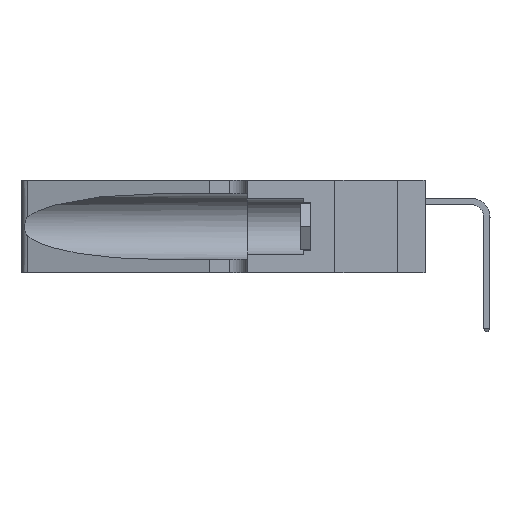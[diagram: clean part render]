
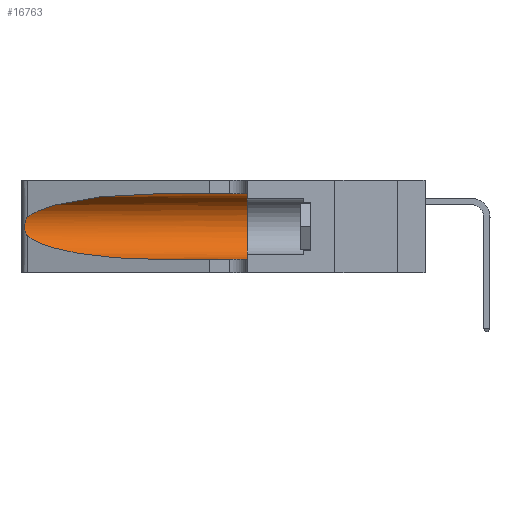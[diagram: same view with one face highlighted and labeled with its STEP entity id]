
A CAD part, left-side view. The second image highlights one B-rep face of the part: STEP entity #16763.
In plain terms, the highlighted cylindrical face has radius 3.308 mm (diameter 6.617 mm), a partial arc.
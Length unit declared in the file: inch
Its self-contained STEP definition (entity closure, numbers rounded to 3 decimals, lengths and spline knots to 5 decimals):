
#260 = CARTESIAN_POINT ( 'NONE',  ( 0.1305, 0.72297, 0.31525 ) ) ;
#301 = CARTESIAN_POINT ( 'NONE',  ( 0.25487, 1.22718, 0.14631 ) ) ;
#3483 = CARTESIAN_POINT ( 'NONE',  ( 0.25639, 1.23184, 0.21858 ) ) ;
#4740 = VERTEX_POINT ( 'NONE', #5156 ) ;
#5156 = CARTESIAN_POINT ( 'NONE',  ( 0.1305, 0.35, 0.31525 ) ) ;
#5335 = LINE ( 'NONE', #23273, #21573 ) ;
#6821 = CARTESIAN_POINT ( 'NONE',  ( 0.25854, 1.2359, 0.20912 ) ) ;
#8259 = EDGE_CURVE ( 'NONE', #13565, #40154, #20886, .T. ) ;
#8665 = CARTESIAN_POINT ( 'NONE',  ( 0.25487, 1.22718, 0.14631 ) ) ;
#10101 = CARTESIAN_POINT ( 'NONE',  ( 0.26075, 1.23896, 0.19203 ) ) ;
#10343 = EDGE_CURVE ( 'NONE', #40500, #4740, #37743, .T. ) ;
#13371 = CARTESIAN_POINT ( 'NONE',  ( 0.26017, 1.23833, 0.17102 ) ) ;
#13480 = CYLINDRICAL_SURFACE ( 'NONE', #17492, 0.13025 ) ;
#13565 = VERTEX_POINT ( 'NONE', #40414 ) ;
#14481 = FACE_OUTER_BOUND ( 'NONE', #26450, .T. ) ;
#14587 = DIRECTION ( 'NONE',  ( 0., 0., -1. ) ) ;
#14667 = CARTESIAN_POINT ( 'NONE',  ( 0.1305, 0.72297, 0.31525 ) ) ;
#15655 = CARTESIAN_POINT ( 'NONE',  ( 0.25487, 1.22718, 0.22369 ) ) ;
#16059 = ORIENTED_EDGE ( 'NONE', *, *, #21133, .T. ) ;
#16588 = CARTESIAN_POINT ( 'NONE',  ( 0.25789, 1.23486, 0.15765 ) ) ;
#16763 = ADVANCED_FACE ( 'NONE', ( #14481 ), #13480, .F. ) ;
#17492 = AXIS2_PLACEMENT_3D ( 'NONE', #21084, #37221, #14587 ) ;
#17765 = CARTESIAN_POINT ( 'NONE',  ( 0.18966, 0.96281, 0.31525 ) ) ;
#18184 = ORIENTED_EDGE ( 'NONE', *, *, #8259, .T. ) ;
#18957 = EDGE_CURVE ( 'NONE', #4740, #27618, #39060, .T. ) ;
#19145 = CARTESIAN_POINT ( 'NONE',  ( 0.1305, 0.35, 0.185 ) ) ;
#19700 = CARTESIAN_POINT ( 'NONE',  ( 0.25487, 1.22718, 0.22369 ) ) ;
#19837 = CARTESIAN_POINT ( 'NONE',  ( 0.25555, 1.22993, 0.14849 ) ) ;
#20022 = DIRECTION ( 'NONE',  ( 0., -1., 0. ) ) ;
#20886 =( BOUNDED_CURVE ( )  B_SPLINE_CURVE ( 3, ( #8665, #24767, #28017, #31290 ),
 .UNSPECIFIED., .F., .T. ) 
 B_SPLINE_CURVE_WITH_KNOTS ( ( 4, 4 ),
 ( 3.44316, 4.71239 ),
 .UNSPECIFIED. ) 
 CURVE ( )  GEOMETRIC_REPRESENTATION_ITEM ( )  RATIONAL_B_SPLINE_CURVE ( ( 1., 0.87, 0.87, 1. ) ) 
 REPRESENTATION_ITEM ( '' )  );
#21084 = CARTESIAN_POINT ( 'NONE',  ( 0.1305, 1.61858, 0.185 ) ) ;
#21133 = EDGE_CURVE ( 'NONE', #40500, #38207, #40310, .T. ) ;
#21573 = VECTOR ( 'NONE', #20022, 39.37008 ) ;
#22254 = DIRECTION ( 'NONE',  ( 0., -1., 0. ) ) ;
#22412 = DIRECTION ( 'NONE',  ( 0., 0., 1. ) ) ;
#22805 = EDGE_CURVE ( 'NONE', #40154, #27618, #5335, .T. ) ;
#22967 = CARTESIAN_POINT ( 'NONE',  ( 0.25555, 1.22994, 0.2215 ) ) ;
#23273 = CARTESIAN_POINT ( 'NONE',  ( 0.1305, 1.61858, 0.05475 ) ) ;
#24256 = CARTESIAN_POINT ( 'NONE',  ( 0.2373, 1.15595, 0.28018 ) ) ;
#24767 = CARTESIAN_POINT ( 'NONE',  ( 0.2373, 1.15595, 0.08982 ) ) ;
#26186 = CARTESIAN_POINT ( 'NONE',  ( 0.25787, 1.23484, 0.2124 ) ) ;
#26450 = EDGE_LOOP ( 'NONE', ( #16059, #27541, #18184, #39934, #29882, #33886 ) ) ;
#27541 = ORIENTED_EDGE ( 'NONE', *, *, #39825, .T. ) ;
#27618 = VERTEX_POINT ( 'NONE', #31024 ) ;
#28017 = CARTESIAN_POINT ( 'NONE',  ( 0.18966, 0.96281, 0.05475 ) ) ;
#29457 = CARTESIAN_POINT ( 'NONE',  ( 0.26018, 1.23835, 0.19895 ) ) ;
#29677 = B_SPLINE_CURVE_WITH_KNOTS ( 'NONE', 3,
 ( #19700, #22967, #3483, #26186, #6821, #29457, #10101, #32696, #13371, #35973, #16588, #39213, #19837, #301 ),
 .UNSPECIFIED., .F., .F.,
 ( 4, 2, 2, 2, 2, 2, 4 ),
 ( 0., 0.00027, 0.00053, 0.00107, 0.0016, 0.00187, 0.00214 ),
 .UNSPECIFIED. ) ;
#29882 = ORIENTED_EDGE ( 'NONE', *, *, #18957, .F. ) ;
#30569 = AXIS2_PLACEMENT_3D ( 'NONE', #19145, #41732, #22412 ) ;
#31024 = CARTESIAN_POINT ( 'NONE',  ( 0.1305, 0.35, 0.05475 ) ) ;
#31290 = CARTESIAN_POINT ( 'NONE',  ( 0.1305, 0.72297, 0.05475 ) ) ;
#32696 = CARTESIAN_POINT ( 'NONE',  ( 0.26075, 1.23896, 0.178 ) ) ;
#33886 = ORIENTED_EDGE ( 'NONE', *, *, #10343, .F. ) ;
#34239 = CARTESIAN_POINT ( 'NONE',  ( 0.1305, 0.72297, 0.05475 ) ) ;
#35128 = CARTESIAN_POINT ( 'NONE',  ( 0.1305, 1.61858, 0.31525 ) ) ;
#35973 = CARTESIAN_POINT ( 'NONE',  ( 0.25856, 1.23593, 0.16098 ) ) ;
#36707 = VECTOR ( 'NONE', #22254, 39.37008 ) ;
#37221 = DIRECTION ( 'NONE',  ( 0., -1., 0. ) ) ;
#37299 = CARTESIAN_POINT ( 'NONE',  ( 0.25487, 1.22718, 0.22369 ) ) ;
#37743 = LINE ( 'NONE', #35128, #36707 ) ;
#38207 = VERTEX_POINT ( 'NONE', #15655 ) ;
#39060 = CIRCLE ( 'NONE', #30569, 0.13025 ) ;
#39213 = CARTESIAN_POINT ( 'NONE',  ( 0.25639, 1.23186, 0.15144 ) ) ;
#39825 = EDGE_CURVE ( 'NONE', #38207, #13565, #29677, .T. ) ;
#39934 = ORIENTED_EDGE ( 'NONE', *, *, #22805, .T. ) ;
#40154 = VERTEX_POINT ( 'NONE', #34239 ) ;
#40310 =( BOUNDED_CURVE ( )  B_SPLINE_CURVE ( 3, ( #14667, #17765, #24256, #37299 ),
 .UNSPECIFIED., .F., .F. ) 
 B_SPLINE_CURVE_WITH_KNOTS ( ( 4, 4 ),
 ( 1.5708, 2.84003 ),
 .UNSPECIFIED. ) 
 CURVE ( )  GEOMETRIC_REPRESENTATION_ITEM ( )  RATIONAL_B_SPLINE_CURVE ( ( 1., 0.87, 0.87, 1. ) ) 
 REPRESENTATION_ITEM ( '' )  );
#40414 = CARTESIAN_POINT ( 'NONE',  ( 0.25487, 1.22718, 0.14631 ) ) ;
#40500 = VERTEX_POINT ( 'NONE', #260 ) ;
#41732 = DIRECTION ( 'NONE',  ( 0., 1., 0. ) ) ;
